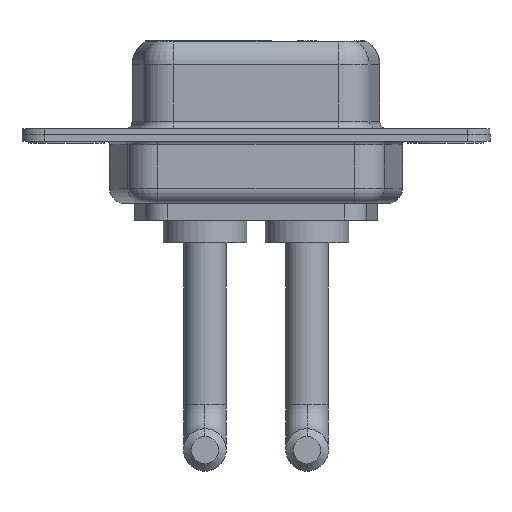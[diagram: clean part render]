
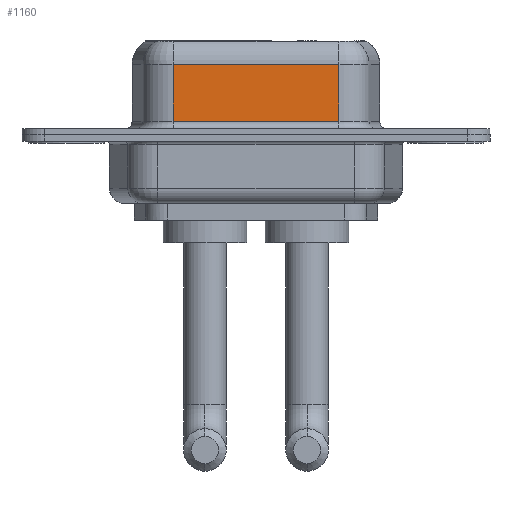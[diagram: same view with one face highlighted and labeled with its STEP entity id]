
A CAD part, front view. The second image highlights one B-rep face of the part: STEP entity #1160.
In plain terms, the highlighted planar face has unit normal (0, -1, 0).
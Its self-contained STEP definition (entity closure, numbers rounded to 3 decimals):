
#1000 = DIRECTION ( 'NONE',  ( 0., 0., -1. ) ) ;
#1130 = EDGE_LOOP ( 'NONE', ( #7478, #7753, #10905, #3248 ) ) ;
#1160 = ADVANCED_FACE ( 'NONE', ( #7744 ), #3183, .F. ) ;
#1869 = DIRECTION ( 'NONE',  ( 1., 0., 0. ) ) ;
#2239 = DIRECTION ( 'NONE',  ( -1., 0., 0. ) ) ;
#2297 = DIRECTION ( 'NONE',  ( 0., 1., 0. ) ) ;
#2361 = CARTESIAN_POINT ( 'NONE',  ( 17.962, -3.95, 6.4 ) ) ;
#2853 = LINE ( 'NONE', #8183, #3473 ) ;
#3163 = EDGE_CURVE ( 'NONE', #8942, #11340, #6013, .T. ) ;
#3183 = PLANE ( 'NONE',  #8789 ) ;
#3248 = ORIENTED_EDGE ( 'NONE', *, *, #8647, .T. ) ;
#3473 = VECTOR ( 'NONE', #1000, 1000. ) ;
#4327 = DIRECTION ( 'NONE',  ( 0., 0., -1. ) ) ;
#4888 = VERTEX_POINT ( 'NONE', #8701 ) ;
#5021 = CARTESIAN_POINT ( 'NONE',  ( 7.038, -3.95, 0.9 ) ) ;
#5529 = VECTOR ( 'NONE', #1869, 1000. ) ;
#5695 = VECTOR ( 'NONE', #4327, 1000. ) ;
#6013 = LINE ( 'NONE', #8538, #6465 ) ;
#6465 = VECTOR ( 'NONE', #6793, 1000. ) ;
#6793 = DIRECTION ( 'NONE',  ( -1., 0., 0. ) ) ;
#7131 = CARTESIAN_POINT ( 'NONE',  ( 17.962, -3.95, 0.9 ) ) ;
#7478 = ORIENTED_EDGE ( 'NONE', *, *, #8581, .F. ) ;
#7744 = FACE_OUTER_BOUND ( 'NONE', #1130, .T. ) ;
#7753 = ORIENTED_EDGE ( 'NONE', *, *, #3163, .T. ) ;
#8183 = CARTESIAN_POINT ( 'NONE',  ( 17.962, -3.95, 6.4 ) ) ;
#8240 = LINE ( 'NONE', #7131, #5529 ) ;
#8273 = VERTEX_POINT ( 'NONE', #5021 ) ;
#8538 = CARTESIAN_POINT ( 'NONE',  ( 17.962, -3.95, 4.65 ) ) ;
#8581 = EDGE_CURVE ( 'NONE', #8942, #4888, #2853, .T. ) ;
#8647 = EDGE_CURVE ( 'NONE', #8273, #4888, #8240, .T. ) ;
#8701 = CARTESIAN_POINT ( 'NONE',  ( 17.962, -3.95, 0.9 ) ) ;
#8789 = AXIS2_PLACEMENT_3D ( 'NONE', #2361, #2297, #2239 ) ;
#8942 = VERTEX_POINT ( 'NONE', #9501 ) ;
#9349 = EDGE_CURVE ( 'NONE', #11340, #8273, #11522, .T. ) ;
#9501 = CARTESIAN_POINT ( 'NONE',  ( 17.962, -3.95, 4.65 ) ) ;
#9831 = CARTESIAN_POINT ( 'NONE',  ( 7.038, -3.95, 6.4 ) ) ;
#10592 = CARTESIAN_POINT ( 'NONE',  ( 7.038, -3.95, 4.65 ) ) ;
#10905 = ORIENTED_EDGE ( 'NONE', *, *, #9349, .T. ) ;
#11340 = VERTEX_POINT ( 'NONE', #10592 ) ;
#11522 = LINE ( 'NONE', #9831, #5695 ) ;
